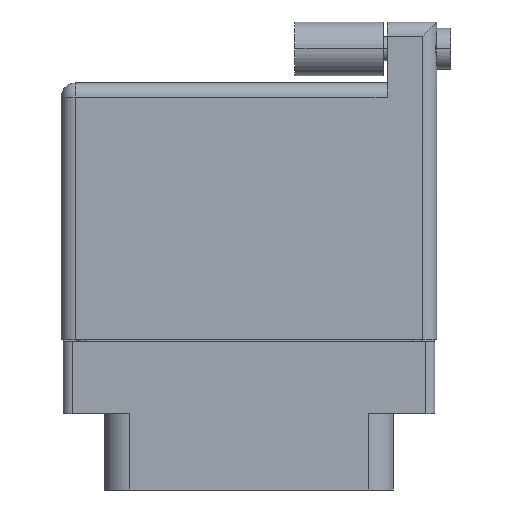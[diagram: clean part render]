
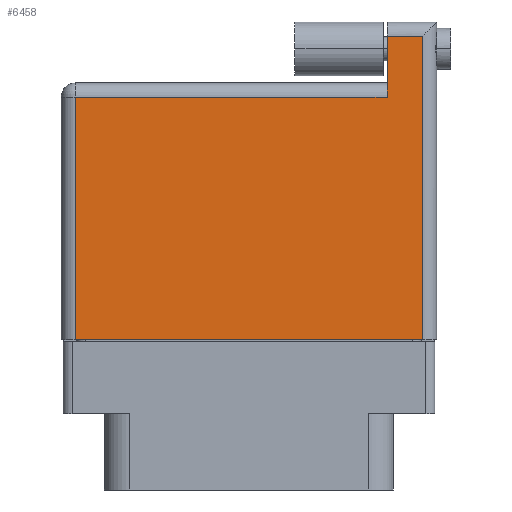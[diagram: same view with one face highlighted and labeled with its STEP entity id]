
A CAD part, front view. The second image highlights one B-rep face of the part: STEP entity #6458.
In plain terms, the highlighted face is planar.
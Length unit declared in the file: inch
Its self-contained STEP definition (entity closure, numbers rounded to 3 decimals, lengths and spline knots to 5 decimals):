
#484 = CARTESIAN_POINT ( 'NONE',  ( -0.6625, 0.97, 0.3575 ) ) ;
#722 = EDGE_CURVE ( 'NONE', #22717, #8673, #11295, .T. ) ;
#2550 = ORIENTED_EDGE ( 'NONE', *, *, #11907, .T. ) ;
#3291 = ORIENTED_EDGE ( 'NONE', *, *, #24480, .T. ) ;
#5519 = CARTESIAN_POINT ( 'NONE',  ( -0.6625, 0.756, 0.3575 ) ) ;
#5920 = LINE ( 'NONE', #8464, #21942 ) ;
#6068 = EDGE_CURVE ( 'NONE', #10570, #12292, #11385, .T. ) ;
#6458 = ADVANCED_FACE ( 'NONE', ( #16956 ), #22939, .F. ) ;
#6822 = LINE ( 'NONE', #23614, #26490 ) ;
#6878 = EDGE_CURVE ( 'NONE', #20006, #11471, #21491, .T. ) ;
#7383 = DIRECTION ( 'NONE',  ( -1., 0., 0. ) ) ;
#8464 = CARTESIAN_POINT ( 'NONE',  ( 0.6125, 1.02, 0.3575 ) ) ;
#8673 = VERTEX_POINT ( 'NONE', #11815 ) ;
#10024 = DIRECTION ( 'NONE',  ( -1., 0., 0. ) ) ;
#10205 = DIRECTION ( 'NONE',  ( 0., 0., -1. ) ) ;
#10570 = VERTEX_POINT ( 'NONE', #17748 ) ;
#11295 = LINE ( 'NONE', #14261, #21117 ) ;
#11385 = LINE ( 'NONE', #484, #15991 ) ;
#11471 = VERTEX_POINT ( 'NONE', #11627 ) ;
#11627 = CARTESIAN_POINT ( 'NONE',  ( -0.6125, 0.756, 0.3575 ) ) ;
#11815 = CARTESIAN_POINT ( 'NONE',  ( 0.6125, -0.1, 0.3575 ) ) ;
#11907 = EDGE_CURVE ( 'NONE', #12292, #20006, #6822, .T. ) ;
#12292 = VERTEX_POINT ( 'NONE', #20742 ) ;
#12819 = DIRECTION ( 'NONE',  ( 0., 1., 0. ) ) ;
#12982 = ORIENTED_EDGE ( 'NONE', *, *, #722, .T. ) ;
#14261 = CARTESIAN_POINT ( 'NONE',  ( -0.6625, -0.1, 0.3575 ) ) ;
#14620 = DIRECTION ( 'NONE',  ( 1., 0., 0. ) ) ;
#15271 = VECTOR ( 'NONE', #20504, 39.37008 ) ;
#15991 = VECTOR ( 'NONE', #7383, 39.37008 ) ;
#16956 = FACE_OUTER_BOUND ( 'NONE', #17795, .T. ) ;
#17096 = ORIENTED_EDGE ( 'NONE', *, *, #6878, .T. ) ;
#17575 = EDGE_CURVE ( 'NONE', #11471, #22717, #25587, .T. ) ;
#17748 = CARTESIAN_POINT ( 'NONE',  ( 0.6125, 0.97, 0.3575 ) ) ;
#17795 = EDGE_LOOP ( 'NONE', ( #12982, #3291, #23609, #2550, #17096, #24935 ) ) ;
#19370 = DIRECTION ( 'NONE',  ( 0., -1., 0. ) ) ;
#20006 = VERTEX_POINT ( 'NONE', #24967 ) ;
#20504 = DIRECTION ( 'NONE',  ( -1., 0., 0. ) ) ;
#20742 = CARTESIAN_POINT ( 'NONE',  ( 0.4875, 0.97, 0.3575 ) ) ;
#21117 = VECTOR ( 'NONE', #14620, 39.37008 ) ;
#21491 = LINE ( 'NONE', #5519, #15271 ) ;
#21942 = VECTOR ( 'NONE', #12819, 39.37008 ) ;
#22571 = CARTESIAN_POINT ( 'NONE',  ( -0.6625, 0.806, 0.3575 ) ) ;
#22717 = VERTEX_POINT ( 'NONE', #23742 ) ;
#22938 = VECTOR ( 'NONE', #24304, 39.37008 ) ;
#22939 = PLANE ( 'NONE',  #25926 ) ;
#23609 = ORIENTED_EDGE ( 'NONE', *, *, #6068, .T. ) ;
#23614 = CARTESIAN_POINT ( 'NONE',  ( 0.4875, 1.02, 0.3575 ) ) ;
#23742 = CARTESIAN_POINT ( 'NONE',  ( -0.6125, -0.1, 0.3575 ) ) ;
#24116 = CARTESIAN_POINT ( 'NONE',  ( -0.6125, -0.1, 0.3575 ) ) ;
#24304 = DIRECTION ( 'NONE',  ( 0., -1., 0. ) ) ;
#24480 = EDGE_CURVE ( 'NONE', #8673, #10570, #5920, .T. ) ;
#24935 = ORIENTED_EDGE ( 'NONE', *, *, #17575, .T. ) ;
#24967 = CARTESIAN_POINT ( 'NONE',  ( 0.4875, 0.756, 0.3575 ) ) ;
#25587 = LINE ( 'NONE', #24116, #22938 ) ;
#25926 = AXIS2_PLACEMENT_3D ( 'NONE', #22571, #10205, #10024 ) ;
#26490 = VECTOR ( 'NONE', #19370, 39.37008 ) ;
